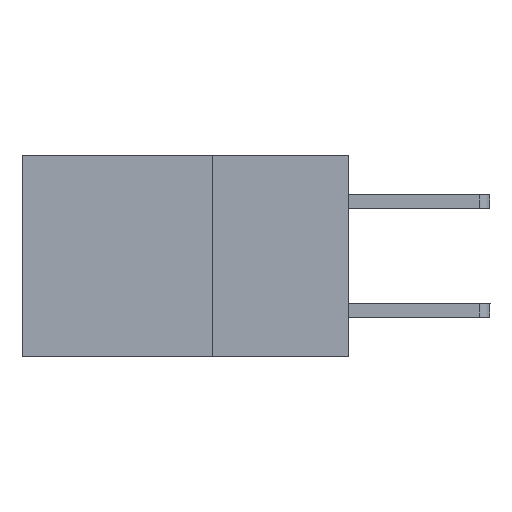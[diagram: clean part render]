
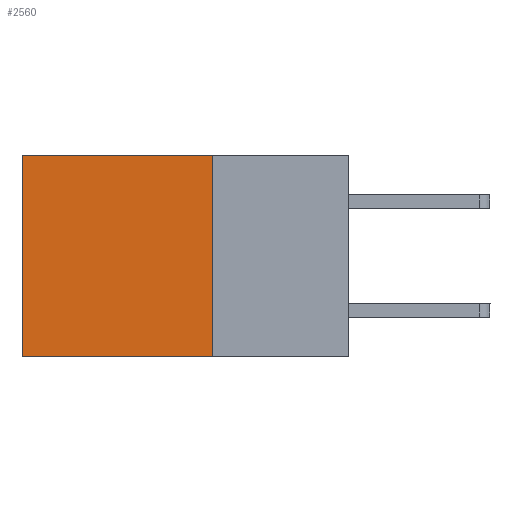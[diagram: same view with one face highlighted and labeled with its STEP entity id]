
A CAD part, left-side view. The second image highlights one B-rep face of the part: STEP entity #2560.
In plain terms, the highlighted planar face has unit normal (-1, 0, 0).
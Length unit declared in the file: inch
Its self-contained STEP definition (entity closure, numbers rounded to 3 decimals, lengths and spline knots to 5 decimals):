
#265 = EDGE_CURVE ( 'NONE', #7277, #7677, #3393, .T. ) ;
#296 = VERTEX_POINT ( 'NONE', #3676 ) ;
#379 = ORIENTED_EDGE ( 'NONE', *, *, #5539, .T. ) ;
#481 = ORIENTED_EDGE ( 'NONE', *, *, #4593, .F. ) ;
#593 = VERTEX_POINT ( 'NONE', #7171 ) ;
#725 = ORIENTED_EDGE ( 'NONE', *, *, #265, .F. ) ;
#858 = ORIENTED_EDGE ( 'NONE', *, *, #5948, .T. ) ;
#1489 = VECTOR ( 'NONE', #5963, 39.37008 ) ;
#1636 = CARTESIAN_POINT ( 'NONE',  ( 0.2615, 0.25, 0. ) ) ;
#1883 = LINE ( 'NONE', #8355, #5219 ) ;
#1961 = EDGE_LOOP ( 'NONE', ( #379, #481, #725, #858 ) ) ;
#2560 = ADVANCED_FACE ( 'NONE', ( #2949 ), #5397, .F. ) ;
#2753 = DIRECTION ( 'NONE',  ( 0., 1., 0. ) ) ;
#2949 = FACE_OUTER_BOUND ( 'NONE', #1961, .T. ) ;
#3251 = LINE ( 'NONE', #3302, #8030 ) ;
#3302 = CARTESIAN_POINT ( 'NONE',  ( 0.2615, 0.25, -0.37 ) ) ;
#3393 = LINE ( 'NONE', #4319, #1489 ) ;
#3676 = CARTESIAN_POINT ( 'NONE',  ( 0.2615, 0.6, 0. ) ) ;
#4319 = CARTESIAN_POINT ( 'NONE',  ( 0.2615, 0.25, -0.37 ) ) ;
#4361 = DIRECTION ( 'NONE',  ( 0., 0., -1. ) ) ;
#4593 = EDGE_CURVE ( 'NONE', #7677, #593, #3251, .T. ) ;
#5219 = VECTOR ( 'NONE', #8332, 39.37008 ) ;
#5397 = PLANE ( 'NONE',  #7273 ) ;
#5539 = EDGE_CURVE ( 'NONE', #296, #593, #1883, .T. ) ;
#5626 = VECTOR ( 'NONE', #6243, 39.37008 ) ;
#5680 = DIRECTION ( 'NONE',  ( 1., 0., 0. ) ) ;
#5948 = EDGE_CURVE ( 'NONE', #7277, #296, #7272, .T. ) ;
#5963 = DIRECTION ( 'NONE',  ( 0., 0., -1. ) ) ;
#6243 = DIRECTION ( 'NONE',  ( 0., 1., 0. ) ) ;
#6564 = CARTESIAN_POINT ( 'NONE',  ( 0.2615, 0.25, 0. ) ) ;
#6925 = CARTESIAN_POINT ( 'NONE',  ( 0.2615, 0.25, -0.37 ) ) ;
#7171 = CARTESIAN_POINT ( 'NONE',  ( 0.2615, 0.6, -0.37 ) ) ;
#7259 = CARTESIAN_POINT ( 'NONE',  ( 0.2615, 0.25, -0.37 ) ) ;
#7272 = LINE ( 'NONE', #6564, #5626 ) ;
#7273 = AXIS2_PLACEMENT_3D ( 'NONE', #6925, #5680, #4361 ) ;
#7277 = VERTEX_POINT ( 'NONE', #1636 ) ;
#7677 = VERTEX_POINT ( 'NONE', #7259 ) ;
#8030 = VECTOR ( 'NONE', #2753, 39.37008 ) ;
#8332 = DIRECTION ( 'NONE',  ( 0., 0., -1. ) ) ;
#8355 = CARTESIAN_POINT ( 'NONE',  ( 0.2615, 0.6, -0.37 ) ) ;
